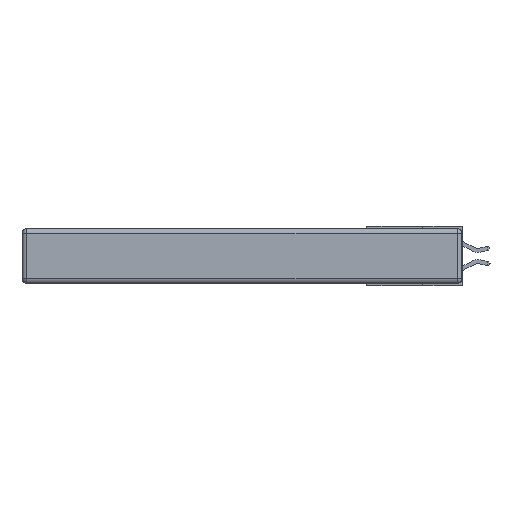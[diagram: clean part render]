
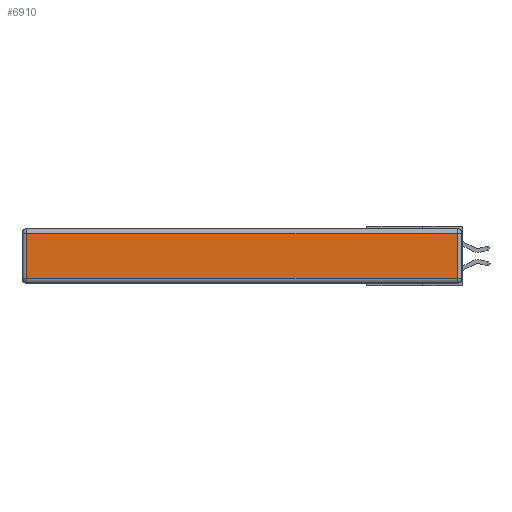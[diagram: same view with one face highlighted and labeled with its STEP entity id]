
A CAD part, left-side view. The second image highlights one B-rep face of the part: STEP entity #6910.
In plain terms, the highlighted planar face has unit normal (-1, 0, 0).
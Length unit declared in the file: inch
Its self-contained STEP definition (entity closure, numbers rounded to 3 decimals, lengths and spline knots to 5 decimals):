
#199 = DIRECTION ( 'NONE',  ( -1., 0., 0. ) ) ;
#562 = FACE_OUTER_BOUND ( 'NONE', #16275, .T. ) ;
#1327 = VECTOR ( 'NONE', #25706, 39.37008 ) ;
#2862 = DIRECTION ( 'NONE',  ( 0., 0., -1. ) ) ;
#3408 = LINE ( 'NONE', #24700, #17478 ) ;
#3721 = CARTESIAN_POINT ( 'NONE',  ( 0., 0.03, -0.313 ) ) ;
#5292 = PLANE ( 'NONE',  #19669 ) ;
#6417 = DIRECTION ( 'NONE',  ( 0., 1., 0. ) ) ;
#6910 = ADVANCED_FACE ( 'NONE', ( #562 ), #5292, .T. ) ;
#7054 = VECTOR ( 'NONE', #2862, 39.37008 ) ;
#10462 = CARTESIAN_POINT ( 'NONE',  ( 0., 0., -0.343 ) ) ;
#11820 = DIRECTION ( 'NONE',  ( 0., -1., 0. ) ) ;
#12905 = ORIENTED_EDGE ( 'NONE', *, *, #23580, .T. ) ;
#12930 = LINE ( 'NONE', #25353, #1327 ) ;
#13622 = EDGE_CURVE ( 'NONE', #29063, #24344, #3408, .T. ) ;
#16275 = EDGE_LOOP ( 'NONE', ( #18581, #12905, #17296, #25564 ) ) ;
#17296 = ORIENTED_EDGE ( 'NONE', *, *, #13622, .T. ) ;
#17478 = VECTOR ( 'NONE', #6417, 39.37008 ) ;
#18249 = DIRECTION ( 'NONE',  ( 0., 0., 1. ) ) ;
#18581 = ORIENTED_EDGE ( 'NONE', *, *, #19935, .T. ) ;
#19639 = EDGE_CURVE ( 'NONE', #24344, #26895, #32347, .T. ) ;
#19669 = AXIS2_PLACEMENT_3D ( 'NONE', #10462, #199, #18249 ) ;
#19935 = EDGE_CURVE ( 'NONE', #26895, #25502, #24391, .T. ) ;
#23567 = VECTOR ( 'NONE', #11820, 39.37008 ) ;
#23580 = EDGE_CURVE ( 'NONE', #25502, #29063, #12930, .T. ) ;
#24344 = VERTEX_POINT ( 'NONE', #30564 ) ;
#24391 = LINE ( 'NONE', #27484, #23567 ) ;
#24700 = CARTESIAN_POINT ( 'NONE',  ( 0., 2.75, -0.03 ) ) ;
#25049 = CARTESIAN_POINT ( 'NONE',  ( 0., 2.72, -0.313 ) ) ;
#25353 = CARTESIAN_POINT ( 'NONE',  ( 0., 0.03, -0.343 ) ) ;
#25502 = VERTEX_POINT ( 'NONE', #3721 ) ;
#25564 = ORIENTED_EDGE ( 'NONE', *, *, #19639, .T. ) ;
#25706 = DIRECTION ( 'NONE',  ( 0., 0., 1. ) ) ;
#26895 = VERTEX_POINT ( 'NONE', #25049 ) ;
#27484 = CARTESIAN_POINT ( 'NONE',  ( 0., 0., -0.313 ) ) ;
#29063 = VERTEX_POINT ( 'NONE', #31094 ) ;
#29255 = CARTESIAN_POINT ( 'NONE',  ( 0., 2.72, -0.343 ) ) ;
#30564 = CARTESIAN_POINT ( 'NONE',  ( 0., 2.72, -0.03 ) ) ;
#31094 = CARTESIAN_POINT ( 'NONE',  ( 0., 0.03, -0.03 ) ) ;
#32347 = LINE ( 'NONE', #29255, #7054 ) ;
